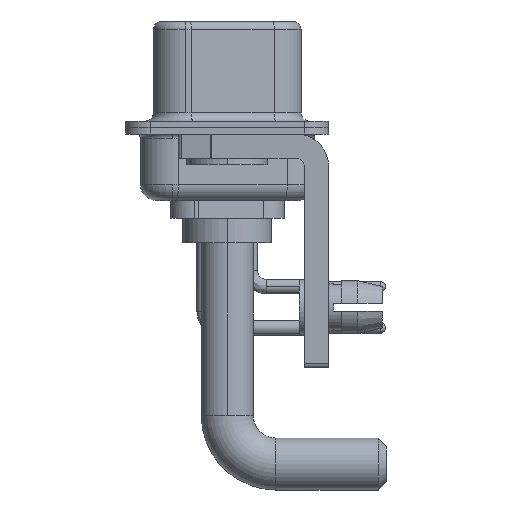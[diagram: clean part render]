
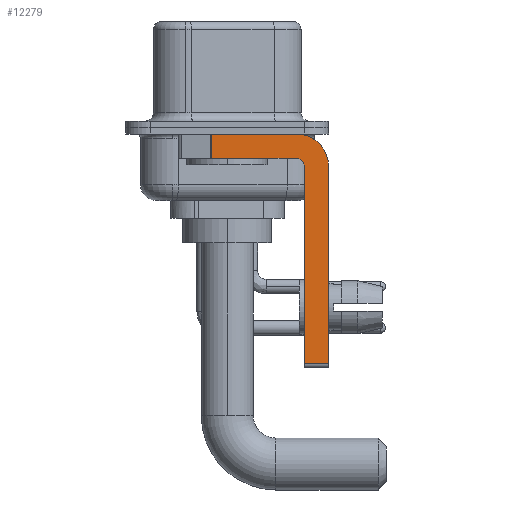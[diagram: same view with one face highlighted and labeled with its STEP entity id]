
A CAD part, left-side view. The second image highlights one B-rep face of the part: STEP entity #12279.
In plain terms, the highlighted planar face has unit normal (-1, 0, 0).
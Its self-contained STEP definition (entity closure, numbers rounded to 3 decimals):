
#430 = VERTEX_POINT ( 'NONE', #24876 ) ;
#613 = CARTESIAN_POINT ( 'NONE',  ( -2.9, -6.25, -14.55 ) ) ;
#1216 = VECTOR ( 'NONE', #10617, 1000. ) ;
#1772 = EDGE_LOOP ( 'NONE', ( #7301, #19309, #24694, #7952, #13814, #4640, #21231, #25062 ) ) ;
#1901 = CARTESIAN_POINT ( 'NONE',  ( -2.9, 3., -0.4 ) ) ;
#2120 = DIRECTION ( 'NONE',  ( 1., 0., 0. ) ) ;
#4030 = LINE ( 'NONE', #8602, #23884 ) ;
#4081 = EDGE_CURVE ( 'NONE', #430, #16373, #13244, .T. ) ;
#4310 = DIRECTION ( 'NONE',  ( 0., 0., -1. ) ) ;
#4464 = DIRECTION ( 'NONE',  ( 0., -1., 0. ) ) ;
#4640 = ORIENTED_EDGE ( 'NONE', *, *, #16228, .T. ) ;
#4780 = CARTESIAN_POINT ( 'NONE',  ( -2.9, -6.25, -2.4 ) ) ;
#6166 = DIRECTION ( 'NONE',  ( 0., -1., 0. ) ) ;
#6645 = CARTESIAN_POINT ( 'NONE',  ( -2.9, -4.25, -0.4 ) ) ;
#6967 = VECTOR ( 'NONE', #6166, 1000. ) ;
#7301 = ORIENTED_EDGE ( 'NONE', *, *, #17136, .F. ) ;
#7593 = AXIS2_PLACEMENT_3D ( 'NONE', #25525, #20519, #12125 ) ;
#7952 = ORIENTED_EDGE ( 'NONE', *, *, #27308, .F. ) ;
#8385 = VERTEX_POINT ( 'NONE', #16865 ) ;
#8602 = CARTESIAN_POINT ( 'NONE',  ( -2.9, -4.25, -14.55 ) ) ;
#8851 = VERTEX_POINT ( 'NONE', #23628 ) ;
#9208 = LINE ( 'NONE', #9492, #16212 ) ;
#9329 = LINE ( 'NONE', #18323, #28368 ) ;
#9492 = CARTESIAN_POINT ( 'NONE',  ( -2.9, -4.25, -1.9 ) ) ;
#9971 = EDGE_CURVE ( 'NONE', #8851, #8385, #9329, .T. ) ;
#10617 = DIRECTION ( 'NONE',  ( 0., 0., -1. ) ) ;
#11743 = VERTEX_POINT ( 'NONE', #6645 ) ;
#12125 = DIRECTION ( 'NONE',  ( 0., 0., -1. ) ) ;
#12279 = ADVANCED_FACE ( 'NONE', ( #22311 ), #22163, .F. ) ;
#13244 = LINE ( 'NONE', #4780, #1216 ) ;
#13563 = CARTESIAN_POINT ( 'NONE',  ( -2.9, -4.25, -1.9 ) ) ;
#13814 = ORIENTED_EDGE ( 'NONE', *, *, #9971, .F. ) ;
#14179 = CIRCLE ( 'NONE', #7593, 2. ) ;
#14477 = VERTEX_POINT ( 'NONE', #27970 ) ;
#15004 = DIRECTION ( 'NONE',  ( 0., 0., -1. ) ) ;
#16106 = DIRECTION ( 'NONE',  ( 0., 0., 1. ) ) ;
#16212 = VECTOR ( 'NONE', #27212, 1000. ) ;
#16228 = EDGE_CURVE ( 'NONE', #8851, #16373, #4030, .T. ) ;
#16373 = VERTEX_POINT ( 'NONE', #613 ) ;
#16835 = VERTEX_POINT ( 'NONE', #13563 ) ;
#16865 = CARTESIAN_POINT ( 'NONE',  ( -2.9, -4.75, -2.4 ) ) ;
#17065 = LINE ( 'NONE', #28298, #28334 ) ;
#17136 = EDGE_CURVE ( 'NONE', #19890, #11743, #26529, .T. ) ;
#17771 = CARTESIAN_POINT ( 'NONE',  ( -2.9, -4.25, -2.4 ) ) ;
#18323 = CARTESIAN_POINT ( 'NONE',  ( -2.9, -4.75, -14.8 ) ) ;
#19309 = ORIENTED_EDGE ( 'NONE', *, *, #22059, .T. ) ;
#19890 = VERTEX_POINT ( 'NONE', #24880 ) ;
#20519 = DIRECTION ( 'NONE',  ( 1., 0., 0. ) ) ;
#20939 = AXIS2_PLACEMENT_3D ( 'NONE', #24521, #2120, #4310 ) ;
#21231 = ORIENTED_EDGE ( 'NONE', *, *, #4081, .F. ) ;
#21457 = EDGE_CURVE ( 'NONE', #11743, #430, #14179, .T. ) ;
#22059 = EDGE_CURVE ( 'NONE', #19890, #14477, #17065, .T. ) ;
#22163 = PLANE ( 'NONE',  #20939 ) ;
#22311 = FACE_OUTER_BOUND ( 'NONE', #1772, .T. ) ;
#23543 = AXIS2_PLACEMENT_3D ( 'NONE', #17771, #28700, #26334 ) ;
#23628 = CARTESIAN_POINT ( 'NONE',  ( -2.9, -4.75, -14.55 ) ) ;
#23884 = VECTOR ( 'NONE', #4464, 1000. ) ;
#24521 = CARTESIAN_POINT ( 'NONE',  ( -2.9, -4.25, -2.4 ) ) ;
#24694 = ORIENTED_EDGE ( 'NONE', *, *, #26076, .F. ) ;
#24876 = CARTESIAN_POINT ( 'NONE',  ( -2.9, -6.25, -2.4 ) ) ;
#24880 = CARTESIAN_POINT ( 'NONE',  ( -2.9, 0.978, -0.4 ) ) ;
#25062 = ORIENTED_EDGE ( 'NONE', *, *, #21457, .F. ) ;
#25525 = CARTESIAN_POINT ( 'NONE',  ( -2.9, -4.25, -2.4 ) ) ;
#26076 = EDGE_CURVE ( 'NONE', #16835, #14477, #9208, .T. ) ;
#26334 = DIRECTION ( 'NONE',  ( 0., 0., 1. ) ) ;
#26529 = LINE ( 'NONE', #1901, #6967 ) ;
#27212 = DIRECTION ( 'NONE',  ( 0., 1., 0. ) ) ;
#27308 = EDGE_CURVE ( 'NONE', #8385, #16835, #28725, .T. ) ;
#27970 = CARTESIAN_POINT ( 'NONE',  ( -2.9, 0.978, -1.9 ) ) ;
#28298 = CARTESIAN_POINT ( 'NONE',  ( -2.9, 0.978, -1.9 ) ) ;
#28334 = VECTOR ( 'NONE', #15004, 1000. ) ;
#28368 = VECTOR ( 'NONE', #16106, 1000. ) ;
#28700 = DIRECTION ( 'NONE',  ( -1., 0., 0. ) ) ;
#28725 = CIRCLE ( 'NONE', #23543, 0.5 ) ;
